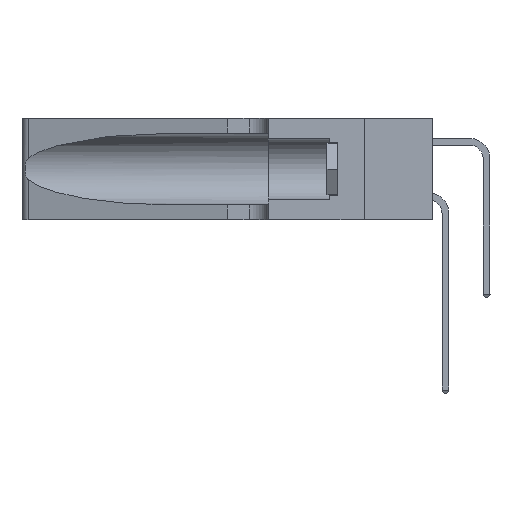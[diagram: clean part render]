
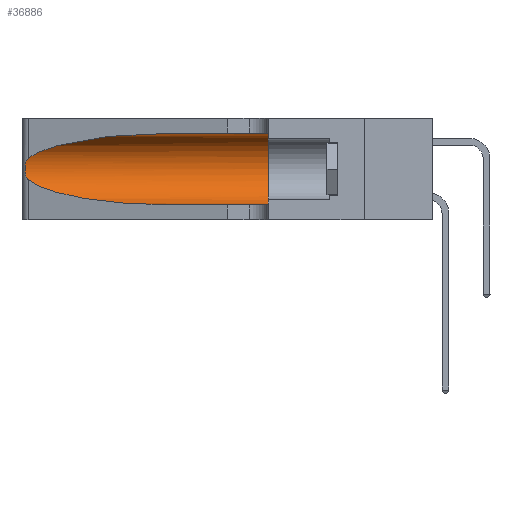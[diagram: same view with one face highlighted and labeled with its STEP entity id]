
A CAD part, left-side view. The second image highlights one B-rep face of the part: STEP entity #36886.
In plain terms, the highlighted cylindrical face has radius 3.308 mm (diameter 6.617 mm), a partial arc.
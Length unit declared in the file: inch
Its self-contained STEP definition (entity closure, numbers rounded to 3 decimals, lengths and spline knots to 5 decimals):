
#268 =( BOUNDED_CURVE ( )  B_SPLINE_CURVE ( 3, ( #4645, #15032, #18474, #42588 ),
 .UNSPECIFIED., .F., .F. ) 
 B_SPLINE_CURVE_WITH_KNOTS ( ( 4, 4 ),
 ( 3.44316, 4.71239 ),
 .UNSPECIFIED. ) 
 CURVE ( )  GEOMETRIC_REPRESENTATION_ITEM ( )  RATIONAL_B_SPLINE_CURVE ( ( 1., 0.87, 0.87, 1. ) ) 
 REPRESENTATION_ITEM ( '' )  );
#374 = VERTEX_POINT ( 'NONE', #2327 ) ;
#1834 = CARTESIAN_POINT ( 'NONE',  ( 0.26018, 1.23835, 0.19895 ) ) ;
#2327 = CARTESIAN_POINT ( 'NONE',  ( 0.25487, 1.22718, 0.22369 ) ) ;
#3074 = EDGE_CURVE ( 'NONE', #24352, #7858, #40552, .T. ) ;
#3594 =( BOUNDED_CURVE ( )  B_SPLINE_CURVE ( 3, ( #27152, #9960, #10108, #34233 ),
 .UNSPECIFIED., .F., .F. ) 
 B_SPLINE_CURVE_WITH_KNOTS ( ( 4, 4 ),
 ( 1.5708, 2.84003 ),
 .UNSPECIFIED. ) 
 CURVE ( )  GEOMETRIC_REPRESENTATION_ITEM ( )  RATIONAL_B_SPLINE_CURVE ( ( 1., 0.87, 0.87, 1. ) ) 
 REPRESENTATION_ITEM ( '' )  );
#4422 = VECTOR ( 'NONE', #18884, 39.37008 ) ;
#4645 = CARTESIAN_POINT ( 'NONE',  ( 0.25487, 1.22718, 0.14631 ) ) ;
#5313 = CARTESIAN_POINT ( 'NONE',  ( 0.26075, 1.23896, 0.178 ) ) ;
#5355 = VERTEX_POINT ( 'NONE', #13784 ) ;
#5373 = CARTESIAN_POINT ( 'NONE',  ( 0.25487, 1.22718, 0.14631 ) ) ;
#7858 = VERTEX_POINT ( 'NONE', #21881 ) ;
#8794 = CARTESIAN_POINT ( 'NONE',  ( 0.25856, 1.23593, 0.16098 ) ) ;
#9960 = CARTESIAN_POINT ( 'NONE',  ( 0.18966, 0.96281, 0.31525 ) ) ;
#10108 = CARTESIAN_POINT ( 'NONE',  ( 0.2373, 1.15595, 0.28018 ) ) ;
#10148 = CARTESIAN_POINT ( 'NONE',  ( 0.1305, 1.61858, 0.31525 ) ) ;
#10852 = VERTEX_POINT ( 'NONE', #5373 ) ;
#12243 = CARTESIAN_POINT ( 'NONE',  ( 0.25639, 1.23186, 0.15144 ) ) ;
#13072 = VECTOR ( 'NONE', #41163, 39.37008 ) ;
#13594 = DIRECTION ( 'NONE',  ( 0., 1., 0. ) ) ;
#13784 = CARTESIAN_POINT ( 'NONE',  ( 0.1305, 0.72297, 0.05475 ) ) ;
#14976 = ORIENTED_EDGE ( 'NONE', *, *, #21681, .F. ) ;
#15032 = CARTESIAN_POINT ( 'NONE',  ( 0.2373, 1.15595, 0.08982 ) ) ;
#15419 = CARTESIAN_POINT ( 'NONE',  ( 0.1305, 1.61858, 0.05475 ) ) ;
#15519 = DIRECTION ( 'NONE',  ( 0., -1., 0. ) ) ;
#15549 = CARTESIAN_POINT ( 'NONE',  ( 0.25487, 1.22718, 0.22369 ) ) ;
#15692 = CARTESIAN_POINT ( 'NONE',  ( 0.25487, 1.22718, 0.14631 ) ) ;
#18474 = CARTESIAN_POINT ( 'NONE',  ( 0.18966, 0.96281, 0.05475 ) ) ;
#18884 = DIRECTION ( 'NONE',  ( 0., -1., 0. ) ) ;
#19014 = CARTESIAN_POINT ( 'NONE',  ( 0.25639, 1.23184, 0.21858 ) ) ;
#21343 = ORIENTED_EDGE ( 'NONE', *, *, #28928, .T. ) ;
#21681 = EDGE_CURVE ( 'NONE', #7858, #21840, #22921, .T. ) ;
#21840 = VERTEX_POINT ( 'NONE', #41891 ) ;
#21881 = CARTESIAN_POINT ( 'NONE',  ( 0.1305, 0.35, 0.31525 ) ) ;
#22451 = DIRECTION ( 'NONE',  ( 0., 0., -1. ) ) ;
#22485 = CARTESIAN_POINT ( 'NONE',  ( 0.25854, 1.2359, 0.20912 ) ) ;
#22921 = CIRCLE ( 'NONE', #35784, 0.13025 ) ;
#22953 = ORIENTED_EDGE ( 'NONE', *, *, #35433, .T. ) ;
#23835 = LINE ( 'NONE', #15419, #4422 ) ;
#24320 = B_SPLINE_CURVE_WITH_KNOTS ( 'NONE', 3,
 ( #15549, #39661, #19014, #43112, #22485, #1834, #25980, #5313, #29471, #8794, #32913, #12243, #36355, #15692 ),
 .UNSPECIFIED., .F., .F.,
 ( 4, 2, 2, 2, 2, 2, 4 ),
 ( 0., 0.00027, 0.00053, 0.00107, 0.0016, 0.00187, 0.00214 ),
 .UNSPECIFIED. ) ;
#24352 = VERTEX_POINT ( 'NONE', #36495 ) ;
#25007 = EDGE_LOOP ( 'NONE', ( #21343, #30776, #22953, #37877, #14976, #39510 ) ) ;
#25980 = CARTESIAN_POINT ( 'NONE',  ( 0.26075, 1.23896, 0.19203 ) ) ;
#27152 = CARTESIAN_POINT ( 'NONE',  ( 0.1305, 0.72297, 0.31525 ) ) ;
#27794 = CYLINDRICAL_SURFACE ( 'NONE', #31833, 0.13025 ) ;
#28928 = EDGE_CURVE ( 'NONE', #24352, #374, #3594, .T. ) ;
#29285 = CARTESIAN_POINT ( 'NONE',  ( 0.1305, 1.61858, 0.185 ) ) ;
#29471 = CARTESIAN_POINT ( 'NONE',  ( 0.26017, 1.23833, 0.17102 ) ) ;
#29992 = FACE_OUTER_BOUND ( 'NONE', #25007, .T. ) ;
#30776 = ORIENTED_EDGE ( 'NONE', *, *, #31147, .T. ) ;
#31147 = EDGE_CURVE ( 'NONE', #374, #10852, #24320, .T. ) ;
#31833 = AXIS2_PLACEMENT_3D ( 'NONE', #29285, #15519, #22451 ) ;
#32913 = CARTESIAN_POINT ( 'NONE',  ( 0.25789, 1.23486, 0.15765 ) ) ;
#34233 = CARTESIAN_POINT ( 'NONE',  ( 0.25487, 1.22718, 0.22369 ) ) ;
#34258 = CARTESIAN_POINT ( 'NONE',  ( 0.1305, 0.35, 0.185 ) ) ;
#35433 = EDGE_CURVE ( 'NONE', #10852, #5355, #268, .T. ) ;
#35784 = AXIS2_PLACEMENT_3D ( 'NONE', #34258, #13594, #37682 ) ;
#36216 = EDGE_CURVE ( 'NONE', #5355, #21840, #23835, .T. ) ;
#36355 = CARTESIAN_POINT ( 'NONE',  ( 0.25555, 1.22993, 0.14849 ) ) ;
#36495 = CARTESIAN_POINT ( 'NONE',  ( 0.1305, 0.72297, 0.31525 ) ) ;
#36886 = ADVANCED_FACE ( 'NONE', ( #29992 ), #27794, .F. ) ;
#37682 = DIRECTION ( 'NONE',  ( 0., 0., 1. ) ) ;
#37877 = ORIENTED_EDGE ( 'NONE', *, *, #36216, .T. ) ;
#39510 = ORIENTED_EDGE ( 'NONE', *, *, #3074, .F. ) ;
#39661 = CARTESIAN_POINT ( 'NONE',  ( 0.25555, 1.22994, 0.2215 ) ) ;
#40552 = LINE ( 'NONE', #10148, #13072 ) ;
#41163 = DIRECTION ( 'NONE',  ( 0., -1., 0. ) ) ;
#41891 = CARTESIAN_POINT ( 'NONE',  ( 0.1305, 0.35, 0.05475 ) ) ;
#42588 = CARTESIAN_POINT ( 'NONE',  ( 0.1305, 0.72297, 0.05475 ) ) ;
#43112 = CARTESIAN_POINT ( 'NONE',  ( 0.25787, 1.23484, 0.2124 ) ) ;
